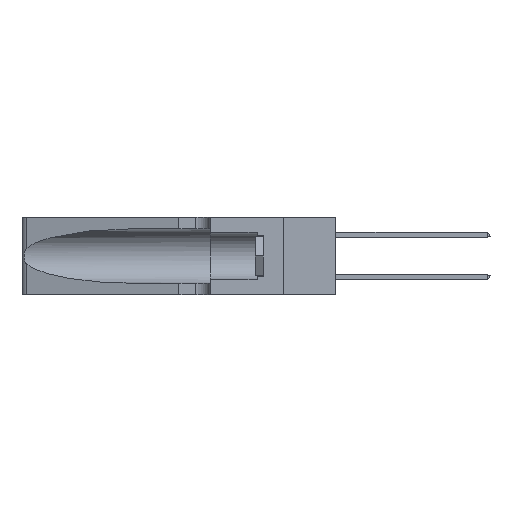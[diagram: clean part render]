
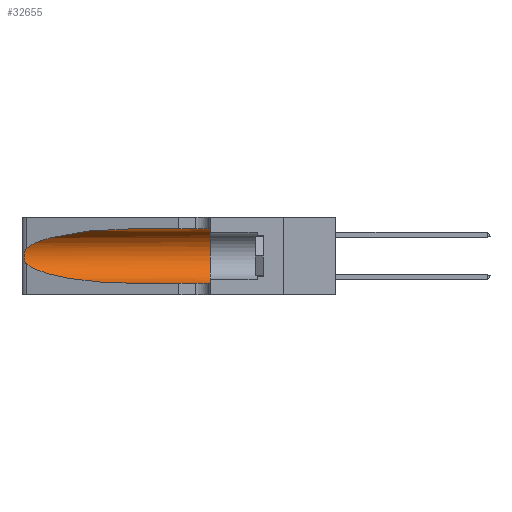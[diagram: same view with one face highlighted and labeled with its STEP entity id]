
A CAD part, left-side view. The second image highlights one B-rep face of the part: STEP entity #32655.
In plain terms, the highlighted cylindrical face has radius 3.308 mm (diameter 6.617 mm), a partial arc.
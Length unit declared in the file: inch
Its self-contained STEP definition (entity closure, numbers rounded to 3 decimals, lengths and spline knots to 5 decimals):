
#17 = CARTESIAN_POINT ( 'NONE',  ( 0.25487, 1.22718, 0.22369 ) ) ;
#160 = CARTESIAN_POINT ( 'NONE',  ( 0.25555, 1.22993, 0.14849 ) ) ;
#1200 = ORIENTED_EDGE ( 'NONE', *, *, #17621, .F. ) ;
#1347 = CARTESIAN_POINT ( 'NONE',  ( 0.18966, 0.96281, 0.05475 ) ) ;
#1375 = CARTESIAN_POINT ( 'NONE',  ( 0.1305, 1.61858, 0.31525 ) ) ;
#2380 = CYLINDRICAL_SURFACE ( 'NONE', #12543, 0.13025 ) ;
#3412 = FACE_OUTER_BOUND ( 'NONE', #15708, .T. ) ;
#3649 = VERTEX_POINT ( 'NONE', #33180 ) ;
#3698 = ORIENTED_EDGE ( 'NONE', *, *, #20723, .T. ) ;
#3708 =( BOUNDED_CURVE ( )  B_SPLINE_CURVE ( 3, ( #22287, #24740, #6434, #28549 ),
 .UNSPECIFIED., .F., .F. ) 
 B_SPLINE_CURVE_WITH_KNOTS ( ( 4, 4 ),
 ( 1.5708, 2.84003 ),
 .UNSPECIFIED. ) 
 CURVE ( )  GEOMETRIC_REPRESENTATION_ITEM ( )  RATIONAL_B_SPLINE_CURVE ( ( 1., 0.87, 0.87, 1. ) ) 
 REPRESENTATION_ITEM ( '' )  );
#4292 = EDGE_CURVE ( 'NONE', #25183, #35383, #35674, .T. ) ;
#6434 = CARTESIAN_POINT ( 'NONE',  ( 0.2373, 1.15595, 0.28018 ) ) ;
#6515 = CARTESIAN_POINT ( 'NONE',  ( 0.25787, 1.23484, 0.2124 ) ) ;
#7756 = LINE ( 'NONE', #38542, #15186 ) ;
#7900 = EDGE_CURVE ( 'NONE', #30915, #3649, #18496, .T. ) ;
#8053 =( BOUNDED_CURVE ( )  B_SPLINE_CURVE ( 3, ( #35944, #10886, #1347, #23661 ),
 .UNSPECIFIED., .F., .F. ) 
 B_SPLINE_CURVE_WITH_KNOTS ( ( 4, 4 ),
 ( 3.44316, 4.71239 ),
 .UNSPECIFIED. ) 
 CURVE ( )  GEOMETRIC_REPRESENTATION_ITEM ( )  RATIONAL_B_SPLINE_CURVE ( ( 1., 0.87, 0.87, 1. ) ) 
 REPRESENTATION_ITEM ( '' )  );
#9614 = CARTESIAN_POINT ( 'NONE',  ( 0.1305, 0.35, 0.185 ) ) ;
#9678 = CARTESIAN_POINT ( 'NONE',  ( 0.1305, 0.72297, 0.05475 ) ) ;
#9728 = CARTESIAN_POINT ( 'NONE',  ( 0.26018, 1.23835, 0.19895 ) ) ;
#10633 = VERTEX_POINT ( 'NONE', #27181 ) ;
#10886 = CARTESIAN_POINT ( 'NONE',  ( 0.2373, 1.15595, 0.08982 ) ) ;
#11398 = ORIENTED_EDGE ( 'NONE', *, *, #7900, .T. ) ;
#12543 = AXIS2_PLACEMENT_3D ( 'NONE', #23190, #19993, #16652 ) ;
#12809 = DIRECTION ( 'NONE',  ( 0., 0., 1. ) ) ;
#12909 = CARTESIAN_POINT ( 'NONE',  ( 0.26075, 1.23896, 0.178 ) ) ;
#14609 = ORIENTED_EDGE ( 'NONE', *, *, #14948, .T. ) ;
#14948 = EDGE_CURVE ( 'NONE', #25183, #30915, #3708, .T. ) ;
#15186 = VECTOR ( 'NONE', #19936, 39.37008 ) ;
#15708 = EDGE_LOOP ( 'NONE', ( #14609, #11398, #22192, #3698, #1200, #22640 ) ) ;
#16097 = CARTESIAN_POINT ( 'NONE',  ( 0.25856, 1.23593, 0.16098 ) ) ;
#16652 = DIRECTION ( 'NONE',  ( 0., 0., -1. ) ) ;
#16840 = CARTESIAN_POINT ( 'NONE',  ( 0.1305, 0.35, 0.31525 ) ) ;
#17621 = EDGE_CURVE ( 'NONE', #35383, #10633, #37955, .T. ) ;
#18496 = B_SPLINE_CURVE_WITH_KNOTS ( 'NONE', 3,
 ( #17, #19166, #25504, #6515, #28614, #9728, #31716, #12909, #34831, #16097, #37921, #19306, #160, #22492 ),
 .UNSPECIFIED., .F., .F.,
 ( 4, 2, 2, 2, 2, 2, 4 ),
 ( 0., 0.00027, 0.00053, 0.00107, 0.0016, 0.00187, 0.00214 ),
 .UNSPECIFIED. ) ;
#19117 = VECTOR ( 'NONE', #29763, 39.37008 ) ;
#19166 = CARTESIAN_POINT ( 'NONE',  ( 0.25555, 1.22994, 0.2215 ) ) ;
#19306 = CARTESIAN_POINT ( 'NONE',  ( 0.25639, 1.23186, 0.15144 ) ) ;
#19936 = DIRECTION ( 'NONE',  ( 0., -1., 0. ) ) ;
#19993 = DIRECTION ( 'NONE',  ( 0., -1., 0. ) ) ;
#20723 = EDGE_CURVE ( 'NONE', #34575, #10633, #7756, .T. ) ;
#22192 = ORIENTED_EDGE ( 'NONE', *, *, #26226, .T. ) ;
#22287 = CARTESIAN_POINT ( 'NONE',  ( 0.1305, 0.72297, 0.31525 ) ) ;
#22492 = CARTESIAN_POINT ( 'NONE',  ( 0.25487, 1.22718, 0.14631 ) ) ;
#22640 = ORIENTED_EDGE ( 'NONE', *, *, #4292, .F. ) ;
#23190 = CARTESIAN_POINT ( 'NONE',  ( 0.1305, 1.61858, 0.185 ) ) ;
#23661 = CARTESIAN_POINT ( 'NONE',  ( 0.1305, 0.72297, 0.05475 ) ) ;
#24740 = CARTESIAN_POINT ( 'NONE',  ( 0.18966, 0.96281, 0.31525 ) ) ;
#25183 = VERTEX_POINT ( 'NONE', #31415 ) ;
#25504 = CARTESIAN_POINT ( 'NONE',  ( 0.25639, 1.23184, 0.21858 ) ) ;
#26226 = EDGE_CURVE ( 'NONE', #3649, #34575, #8053, .T. ) ;
#26769 = AXIS2_PLACEMENT_3D ( 'NONE', #9614, #31598, #12809 ) ;
#27181 = CARTESIAN_POINT ( 'NONE',  ( 0.1305, 0.35, 0.05475 ) ) ;
#28549 = CARTESIAN_POINT ( 'NONE',  ( 0.25487, 1.22718, 0.22369 ) ) ;
#28614 = CARTESIAN_POINT ( 'NONE',  ( 0.25854, 1.2359, 0.20912 ) ) ;
#29763 = DIRECTION ( 'NONE',  ( 0., -1., 0. ) ) ;
#30915 = VERTEX_POINT ( 'NONE', #40068 ) ;
#31415 = CARTESIAN_POINT ( 'NONE',  ( 0.1305, 0.72297, 0.31525 ) ) ;
#31598 = DIRECTION ( 'NONE',  ( 0., 1., 0. ) ) ;
#31716 = CARTESIAN_POINT ( 'NONE',  ( 0.26075, 1.23896, 0.19203 ) ) ;
#32655 = ADVANCED_FACE ( 'NONE', ( #3412 ), #2380, .F. ) ;
#33180 = CARTESIAN_POINT ( 'NONE',  ( 0.25487, 1.22718, 0.14631 ) ) ;
#34575 = VERTEX_POINT ( 'NONE', #9678 ) ;
#34831 = CARTESIAN_POINT ( 'NONE',  ( 0.26017, 1.23833, 0.17102 ) ) ;
#35383 = VERTEX_POINT ( 'NONE', #16840 ) ;
#35674 = LINE ( 'NONE', #1375, #19117 ) ;
#35944 = CARTESIAN_POINT ( 'NONE',  ( 0.25487, 1.22718, 0.14631 ) ) ;
#37921 = CARTESIAN_POINT ( 'NONE',  ( 0.25789, 1.23486, 0.15765 ) ) ;
#37955 = CIRCLE ( 'NONE', #26769, 0.13025 ) ;
#38542 = CARTESIAN_POINT ( 'NONE',  ( 0.1305, 1.61858, 0.05475 ) ) ;
#40068 = CARTESIAN_POINT ( 'NONE',  ( 0.25487, 1.22718, 0.22369 ) ) ;
